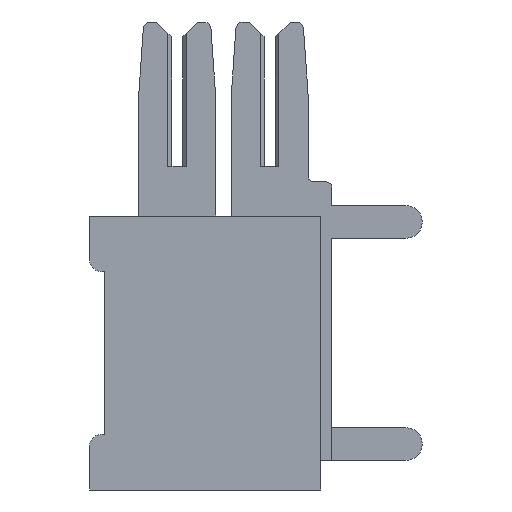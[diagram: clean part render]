
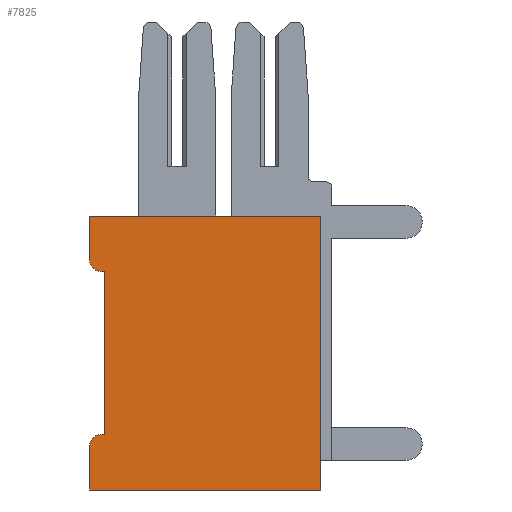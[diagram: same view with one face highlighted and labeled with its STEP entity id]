
A CAD part, left-side view. The second image highlights one B-rep face of the part: STEP entity #7825.
In plain terms, the highlighted planar face has unit normal (-1, 0, 0).
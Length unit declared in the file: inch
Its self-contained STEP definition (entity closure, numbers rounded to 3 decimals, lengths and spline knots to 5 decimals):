
#156 = VERTEX_POINT ( 'NONE', #8269 ) ;
#230 = VERTEX_POINT ( 'NONE', #2108 ) ;
#525 = VERTEX_POINT ( 'NONE', #1146 ) ;
#677 = AXIS2_PLACEMENT_3D ( 'NONE', #7407, #10170, #8353 ) ;
#738 = CARTESIAN_POINT ( 'NONE',  ( 0., 0.312, -0.075 ) ) ;
#774 = VERTEX_POINT ( 'NONE', #9587 ) ;
#784 = DIRECTION ( 'NONE',  ( 0., 0., 1. ) ) ;
#880 = EDGE_CURVE ( 'NONE', #230, #5821, #6274, .T. ) ;
#883 = EDGE_CURVE ( 'NONE', #11618, #2884, #7142, .T. ) ;
#898 = CARTESIAN_POINT ( 'NONE',  ( 0., 0.312, -0.37 ) ) ;
#1020 = CARTESIAN_POINT ( 'NONE',  ( 0., 0., -0.37 ) ) ;
#1146 = CARTESIAN_POINT ( 'NONE',  ( 0., 0.292, -0.295 ) ) ;
#1166 = LINE ( 'NONE', #5757, #7740 ) ;
#1187 = ORIENTED_EDGE ( 'NONE', *, *, #880, .F. ) ;
#1573 = VECTOR ( 'NONE', #5536, 39.37008 ) ;
#1826 = EDGE_CURVE ( 'NONE', #5752, #525, #6103, .T. ) ;
#2098 = VECTOR ( 'NONE', #3947, 39.37008 ) ;
#2108 = CARTESIAN_POINT ( 'NONE',  ( 0., 0.312, -0.37 ) ) ;
#2546 = ORIENTED_EDGE ( 'NONE', *, *, #5012, .T. ) ;
#2696 = DIRECTION ( 'NONE',  ( 0., 1., 0. ) ) ;
#2860 = CARTESIAN_POINT ( 'NONE',  ( 0., 0., 0. ) ) ;
#2884 = VERTEX_POINT ( 'NONE', #10661 ) ;
#3095 = EDGE_CURVE ( 'NONE', #525, #11618, #1166, .T. ) ;
#3638 = AXIS2_PLACEMENT_3D ( 'NONE', #1020, #3782, #9665 ) ;
#3782 = DIRECTION ( 'NONE',  ( -1., 0., 0. ) ) ;
#3820 = CARTESIAN_POINT ( 'NONE',  ( 0., 0.297, -0.295 ) ) ;
#3866 = CARTESIAN_POINT ( 'NONE',  ( 0., 0.312, -0.295 ) ) ;
#3873 = EDGE_CURVE ( 'NONE', #774, #156, #8014, .T. ) ;
#3947 = DIRECTION ( 'NONE',  ( 0., -1., 0. ) ) ;
#4475 = AXIS2_PLACEMENT_3D ( 'NONE', #4555, #5314, #6197 ) ;
#4555 = CARTESIAN_POINT ( 'NONE',  ( 0., 0.297, -0.31 ) ) ;
#4584 = CARTESIAN_POINT ( 'NONE',  ( 0., 0.292, -0.075 ) ) ;
#4854 = EDGE_CURVE ( 'NONE', #5752, #5821, #6854, .T. ) ;
#4906 = ORIENTED_EDGE ( 'NONE', *, *, #5019, .T. ) ;
#5012 = EDGE_CURVE ( 'NONE', #5943, #6648, #6276, .T. ) ;
#5019 = EDGE_CURVE ( 'NONE', #774, #2884, #9435, .T. ) ;
#5296 = ORIENTED_EDGE ( 'NONE', *, *, #883, .F. ) ;
#5314 = DIRECTION ( 'NONE',  ( -1., 0., 0. ) ) ;
#5536 = DIRECTION ( 'NONE',  ( 0., 0., 1. ) ) ;
#5571 = ORIENTED_EDGE ( 'NONE', *, *, #4854, .T. ) ;
#5752 = VERTEX_POINT ( 'NONE', #3820 ) ;
#5757 = CARTESIAN_POINT ( 'NONE',  ( 0., 0.292, -0.295 ) ) ;
#5821 = VERTEX_POINT ( 'NONE', #10190 ) ;
#5943 = VERTEX_POINT ( 'NONE', #7618 ) ;
#6070 = ORIENTED_EDGE ( 'NONE', *, *, #3873, .F. ) ;
#6103 = LINE ( 'NONE', #3866, #2098 ) ;
#6197 = DIRECTION ( 'NONE',  ( 0., 0., 1. ) ) ;
#6274 = LINE ( 'NONE', #8046, #11568 ) ;
#6276 = LINE ( 'NONE', #9201, #10290 ) ;
#6599 = ORIENTED_EDGE ( 'NONE', *, *, #11525, .T. ) ;
#6648 = VERTEX_POINT ( 'NONE', #2860 ) ;
#6854 = CIRCLE ( 'NONE', #4475, 0.015 ) ;
#7142 = LINE ( 'NONE', #738, #9433 ) ;
#7407 = CARTESIAN_POINT ( 'NONE',  ( 0., 0.297, -0.06 ) ) ;
#7618 = CARTESIAN_POINT ( 'NONE',  ( 0., 0., -0.37 ) ) ;
#7740 = VECTOR ( 'NONE', #8443, 39.37008 ) ;
#7793 = FACE_OUTER_BOUND ( 'NONE', #8862, .T. ) ;
#7825 = ADVANCED_FACE ( 'NONE', ( #7793 ), #11702, .T. ) ;
#8014 = LINE ( 'NONE', #898, #1573 ) ;
#8046 = CARTESIAN_POINT ( 'NONE',  ( 0., 0.312, -0.37 ) ) ;
#8269 = CARTESIAN_POINT ( 'NONE',  ( 0., 0.312, 0. ) ) ;
#8353 = DIRECTION ( 'NONE',  ( 0., 0., 1. ) ) ;
#8443 = DIRECTION ( 'NONE',  ( 0., 0., 1. ) ) ;
#8769 = ORIENTED_EDGE ( 'NONE', *, *, #10988, .F. ) ;
#8853 = CARTESIAN_POINT ( 'NONE',  ( 0., 0., 0. ) ) ;
#8862 = EDGE_LOOP ( 'NONE', ( #6070, #4906, #5296, #11391, #11643, #5571, #1187, #6599, #2546, #8769 ) ) ;
#9201 = CARTESIAN_POINT ( 'NONE',  ( 0., 0., -0.37 ) ) ;
#9380 = LINE ( 'NONE', #8853, #10515 ) ;
#9433 = VECTOR ( 'NONE', #2696, 39.37008 ) ;
#9435 = CIRCLE ( 'NONE', #677, 0.015 ) ;
#9587 = CARTESIAN_POINT ( 'NONE',  ( 0., 0.312, -0.06 ) ) ;
#9665 = DIRECTION ( 'NONE',  ( 0., 0., 1. ) ) ;
#10092 = DIRECTION ( 'NONE',  ( 0., 0., 1. ) ) ;
#10170 = DIRECTION ( 'NONE',  ( -1., 0., 0. ) ) ;
#10190 = CARTESIAN_POINT ( 'NONE',  ( 0., 0.312, -0.31 ) ) ;
#10290 = VECTOR ( 'NONE', #10092, 39.37008 ) ;
#10515 = VECTOR ( 'NONE', #10656, 39.37008 ) ;
#10656 = DIRECTION ( 'NONE',  ( 0., -1., 0. ) ) ;
#10661 = CARTESIAN_POINT ( 'NONE',  ( 0., 0.297, -0.075 ) ) ;
#10743 = DIRECTION ( 'NONE',  ( 0., -1., 0. ) ) ;
#10988 = EDGE_CURVE ( 'NONE', #156, #6648, #9380, .T. ) ;
#11357 = LINE ( 'NONE', #11673, #11510 ) ;
#11391 = ORIENTED_EDGE ( 'NONE', *, *, #3095, .F. ) ;
#11510 = VECTOR ( 'NONE', #10743, 39.37008 ) ;
#11525 = EDGE_CURVE ( 'NONE', #230, #5943, #11357, .T. ) ;
#11568 = VECTOR ( 'NONE', #784, 39.37008 ) ;
#11618 = VERTEX_POINT ( 'NONE', #4584 ) ;
#11643 = ORIENTED_EDGE ( 'NONE', *, *, #1826, .F. ) ;
#11673 = CARTESIAN_POINT ( 'NONE',  ( 0., 0., -0.37 ) ) ;
#11702 = PLANE ( 'NONE',  #3638 ) ;
